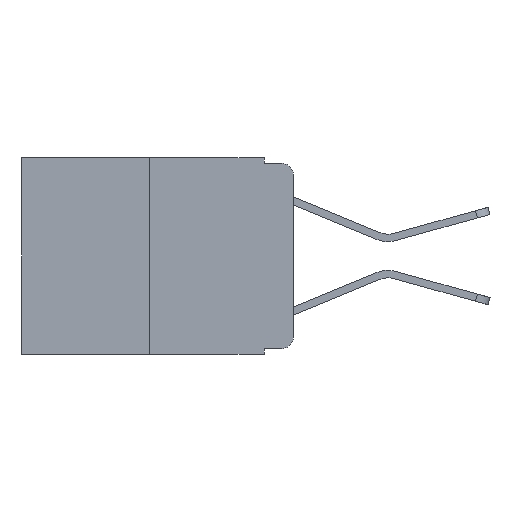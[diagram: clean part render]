
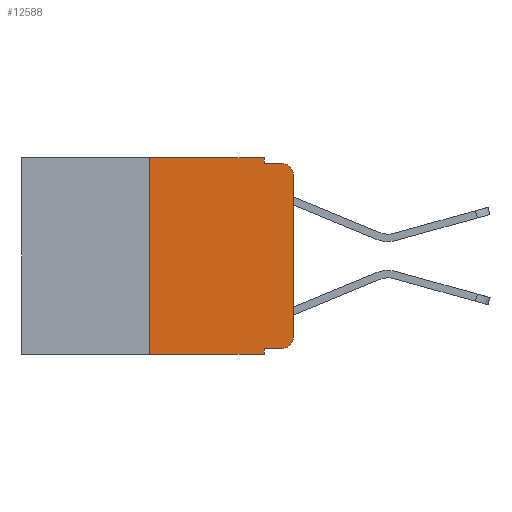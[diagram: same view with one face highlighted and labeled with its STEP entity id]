
A CAD part, left-side view. The second image highlights one B-rep face of the part: STEP entity #12588.
In plain terms, the highlighted planar face has unit normal (-1, 0, 0).
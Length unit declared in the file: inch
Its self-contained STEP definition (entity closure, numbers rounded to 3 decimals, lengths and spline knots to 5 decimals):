
#161 = DIRECTION ( 'NONE',  ( 0., 0., -1. ) ) ;
#313 = CARTESIAN_POINT ( 'NONE',  ( 0., 0.02, -0.03 ) ) ;
#586 = EDGE_CURVE ( 'NONE', #10091, #4077, #2082, .T. ) ;
#998 = VERTEX_POINT ( 'NONE', #2129 ) ;
#1048 = CARTESIAN_POINT ( 'NONE',  ( 0., 0.473, 0. ) ) ;
#1209 = ORIENTED_EDGE ( 'NONE', *, *, #7052, .F. ) ;
#1305 = VERTEX_POINT ( 'NONE', #8961 ) ;
#1321 = LINE ( 'NONE', #3764, #10602 ) ;
#1344 = EDGE_LOOP ( 'NONE', ( #14444, #11618, #10442, #1209, #13637, #7677, #2258, #6984, #14160, #8015 ) ) ;
#1444 = CIRCLE ( 'NONE', #6540, 0.02 ) ;
#1542 = DIRECTION ( 'NONE',  ( 0., -1., 0. ) ) ;
#1855 = CARTESIAN_POINT ( 'NONE',  ( 0., 0.02, -0.01 ) ) ;
#2061 = LINE ( 'NONE', #12450, #3964 ) ;
#2082 = CIRCLE ( 'NONE', #14364, 0.02 ) ;
#2129 = CARTESIAN_POINT ( 'NONE',  ( 0., 0.051, -0.343 ) ) ;
#2150 = DIRECTION ( 'NONE',  ( 0., 0., -1. ) ) ;
#2258 = ORIENTED_EDGE ( 'NONE', *, *, #11780, .T. ) ;
#2481 = VERTEX_POINT ( 'NONE', #15366 ) ;
#2617 = VERTEX_POINT ( 'NONE', #12042 ) ;
#3335 = DIRECTION ( 'NONE',  ( 0., 0., -1. ) ) ;
#3455 = CARTESIAN_POINT ( 'NONE',  ( 0., 0., -0.03 ) ) ;
#3477 = VERTEX_POINT ( 'NONE', #4448 ) ;
#3764 = CARTESIAN_POINT ( 'NONE',  ( 0., 0.051, -0.333 ) ) ;
#3964 = VECTOR ( 'NONE', #7565, 39.37008 ) ;
#3977 = DIRECTION ( 'NONE',  ( 0., -1., 0. ) ) ;
#4003 = CARTESIAN_POINT ( 'NONE',  ( 0., 0.25, 0. ) ) ;
#4077 = VERTEX_POINT ( 'NONE', #1855 ) ;
#4448 = CARTESIAN_POINT ( 'NONE',  ( 0., 0.02, -0.333 ) ) ;
#4819 = LINE ( 'NONE', #9198, #8990 ) ;
#4848 = CARTESIAN_POINT ( 'NONE',  ( 0., 0.051, 0. ) ) ;
#5163 = EDGE_CURVE ( 'NONE', #3477, #9078, #1444, .T. ) ;
#5579 = VERTEX_POINT ( 'NONE', #5741 ) ;
#5741 = CARTESIAN_POINT ( 'NONE',  ( 0., 0.051, 0. ) ) ;
#5941 = EDGE_CURVE ( 'NONE', #13078, #5579, #4819, .T. ) ;
#5971 = DIRECTION ( 'NONE',  ( -1., 0., 0. ) ) ;
#6409 = VECTOR ( 'NONE', #12236, 39.37008 ) ;
#6540 = AXIS2_PLACEMENT_3D ( 'NONE', #13128, #5971, #2150 ) ;
#6781 = CARTESIAN_POINT ( 'NONE',  ( 0., 0.051, 0. ) ) ;
#6873 = VECTOR ( 'NONE', #15245, 39.37008 ) ;
#6984 = ORIENTED_EDGE ( 'NONE', *, *, #9230, .F. ) ;
#7052 = EDGE_CURVE ( 'NONE', #5579, #1305, #14590, .T. ) ;
#7151 = CARTESIAN_POINT ( 'NONE',  ( 0., 0.051, -0.01 ) ) ;
#7261 = DIRECTION ( 'NONE',  ( 0., -1., 0. ) ) ;
#7454 = DIRECTION ( 'NONE',  ( -1., 0., 0. ) ) ;
#7565 = DIRECTION ( 'NONE',  ( 0., 0., 1. ) ) ;
#7677 = ORIENTED_EDGE ( 'NONE', *, *, #14149, .F. ) ;
#8015 = ORIENTED_EDGE ( 'NONE', *, *, #5163, .T. ) ;
#8262 = VECTOR ( 'NONE', #12552, 39.37008 ) ;
#8585 = EDGE_CURVE ( 'NONE', #2481, #3477, #1321, .T. ) ;
#8961 = CARTESIAN_POINT ( 'NONE',  ( 0., 0.051, -0.01 ) ) ;
#8990 = VECTOR ( 'NONE', #15181, 39.37008 ) ;
#9078 = VERTEX_POINT ( 'NONE', #13143 ) ;
#9198 = CARTESIAN_POINT ( 'NONE',  ( 0., 0.473, 0. ) ) ;
#9230 = EDGE_CURVE ( 'NONE', #2481, #998, #9632, .T. ) ;
#9337 = VECTOR ( 'NONE', #7261, 39.37008 ) ;
#9390 = EDGE_CURVE ( 'NONE', #9078, #10091, #2061, .T. ) ;
#9526 = DIRECTION ( 'NONE',  ( 1., 0., 0. ) ) ;
#9632 = LINE ( 'NONE', #4848, #6409 ) ;
#10091 = VERTEX_POINT ( 'NONE', #3455 ) ;
#10381 = FACE_OUTER_BOUND ( 'NONE', #1344, .T. ) ;
#10442 = ORIENTED_EDGE ( 'NONE', *, *, #15300, .F. ) ;
#10591 = VECTOR ( 'NONE', #1542, 39.37008 ) ;
#10602 = VECTOR ( 'NONE', #3977, 39.37008 ) ;
#10962 = CARTESIAN_POINT ( 'NONE',  ( 0., 0.473, -0.343 ) ) ;
#11618 = ORIENTED_EDGE ( 'NONE', *, *, #586, .T. ) ;
#11780 = EDGE_CURVE ( 'NONE', #2617, #998, #14151, .T. ) ;
#11859 = AXIS2_PLACEMENT_3D ( 'NONE', #1048, #9526, #3335 ) ;
#12042 = CARTESIAN_POINT ( 'NONE',  ( 0., 0.25, -0.343 ) ) ;
#12236 = DIRECTION ( 'NONE',  ( 0., 0., -1. ) ) ;
#12450 = CARTESIAN_POINT ( 'NONE',  ( 0., 0., 0. ) ) ;
#12523 = LINE ( 'NONE', #7151, #9337 ) ;
#12552 = DIRECTION ( 'NONE',  ( 0., 0., 1. ) ) ;
#12588 = ADVANCED_FACE ( 'NONE', ( #10381 ), #15547, .F. ) ;
#13078 = VERTEX_POINT ( 'NONE', #15268 ) ;
#13128 = CARTESIAN_POINT ( 'NONE',  ( 0., 0.02, -0.313 ) ) ;
#13143 = CARTESIAN_POINT ( 'NONE',  ( 0., 0., -0.313 ) ) ;
#13508 = LINE ( 'NONE', #4003, #8262 ) ;
#13637 = ORIENTED_EDGE ( 'NONE', *, *, #5941, .F. ) ;
#14149 = EDGE_CURVE ( 'NONE', #2617, #13078, #13508, .T. ) ;
#14151 = LINE ( 'NONE', #10962, #10591 ) ;
#14160 = ORIENTED_EDGE ( 'NONE', *, *, #8585, .T. ) ;
#14364 = AXIS2_PLACEMENT_3D ( 'NONE', #313, #7454, #161 ) ;
#14444 = ORIENTED_EDGE ( 'NONE', *, *, #9390, .T. ) ;
#14590 = LINE ( 'NONE', #6781, #6873 ) ;
#15181 = DIRECTION ( 'NONE',  ( 0., -1., 0. ) ) ;
#15245 = DIRECTION ( 'NONE',  ( 0., 0., -1. ) ) ;
#15268 = CARTESIAN_POINT ( 'NONE',  ( 0., 0.25, 0. ) ) ;
#15300 = EDGE_CURVE ( 'NONE', #1305, #4077, #12523, .T. ) ;
#15366 = CARTESIAN_POINT ( 'NONE',  ( 0., 0.051, -0.333 ) ) ;
#15547 = PLANE ( 'NONE',  #11859 ) ;
